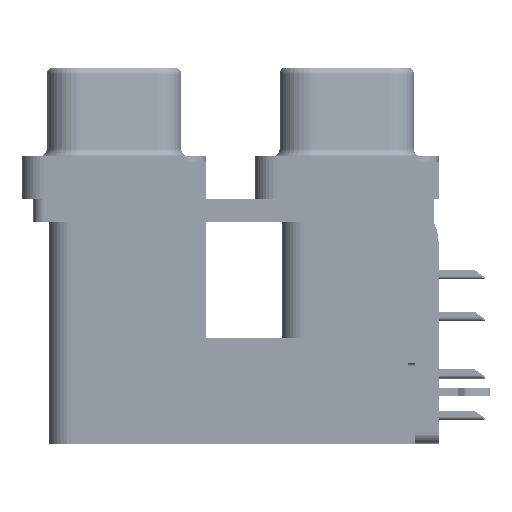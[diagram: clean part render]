
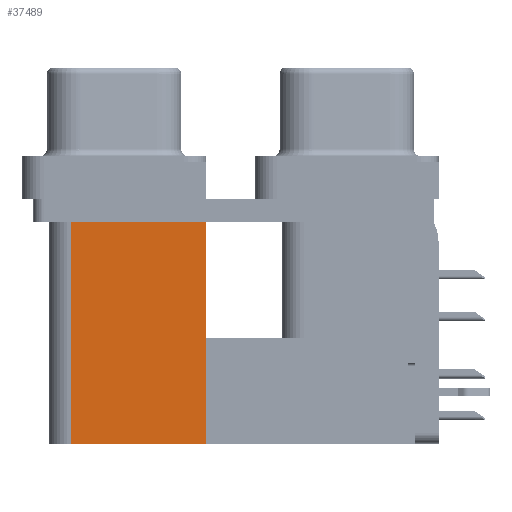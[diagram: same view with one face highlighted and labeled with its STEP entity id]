
A CAD part, left-side view. The second image highlights one B-rep face of the part: STEP entity #37489.
In plain terms, the highlighted planar face has unit normal (-1, 0, 0).
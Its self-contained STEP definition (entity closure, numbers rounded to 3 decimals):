
#683 = DIRECTION ( 'NONE',  ( 0., 1., 0. ) ) ;
#1632 = VECTOR ( 'NONE', #683, 1000. ) ;
#2077 = LINE ( 'NONE', #22358, #21959 ) ;
#6823 = ORIENTED_EDGE ( 'NONE', *, *, #8162, .T. ) ;
#7045 = EDGE_CURVE ( 'NONE', #44615, #36354, #29477, .T. ) ;
#8162 = EDGE_CURVE ( 'NONE', #44615, #46907, #8947, .T. ) ;
#8218 = CARTESIAN_POINT ( 'NONE',  ( 3.79, 9.6, -19.2 ) ) ;
#8947 = LINE ( 'NONE', #44654, #21041 ) ;
#10580 = CARTESIAN_POINT ( 'NONE',  ( 3.79, 18.8, -19.2 ) ) ;
#11832 = AXIS2_PLACEMENT_3D ( 'NONE', #8218, #40719, #20476 ) ;
#12239 = FACE_OUTER_BOUND ( 'NONE', #30949, .T. ) ;
#14027 = CARTESIAN_POINT ( 'NONE',  ( 3.79, 9.6, -19.2 ) ) ;
#14357 = ORIENTED_EDGE ( 'NONE', *, *, #27349, .F. ) ;
#18900 = DIRECTION ( 'NONE',  ( 0., 0., 1. ) ) ;
#19880 = DIRECTION ( 'NONE',  ( 0., 1., 0. ) ) ;
#20476 = DIRECTION ( 'NONE',  ( 0., 0., -1. ) ) ;
#21041 = VECTOR ( 'NONE', #24153, 1000. ) ;
#21281 = ORIENTED_EDGE ( 'NONE', *, *, #7045, .F. ) ;
#21959 = VECTOR ( 'NONE', #18900, 1000. ) ;
#22358 = CARTESIAN_POINT ( 'NONE',  ( 3.79, 18.8, -19.2 ) ) ;
#24153 = DIRECTION ( 'NONE',  ( 0., 0., 1. ) ) ;
#27349 = EDGE_CURVE ( 'NONE', #36354, #45209, #2077, .T. ) ;
#27851 = EDGE_CURVE ( 'NONE', #46907, #45209, #49165, .T. ) ;
#28479 = PLANE ( 'NONE',  #11832 ) ;
#29477 = LINE ( 'NONE', #14027, #1632 ) ;
#30949 = EDGE_LOOP ( 'NONE', ( #37202, #14357, #21281, #6823 ) ) ;
#35881 = CARTESIAN_POINT ( 'NONE',  ( 3.79, 9.6, -19.2 ) ) ;
#36354 = VERTEX_POINT ( 'NONE', #10580 ) ;
#37202 = ORIENTED_EDGE ( 'NONE', *, *, #27851, .T. ) ;
#37489 = ADVANCED_FACE ( 'NONE', ( #12239 ), #28479, .F. ) ;
#37788 = CARTESIAN_POINT ( 'NONE',  ( 3.79, 9.6, -2.5 ) ) ;
#40719 = DIRECTION ( 'NONE',  ( 1., 0., 0. ) ) ;
#40855 = CARTESIAN_POINT ( 'NONE',  ( 3.79, 18.8, -2.5 ) ) ;
#43852 = CARTESIAN_POINT ( 'NONE',  ( 3.79, 9.6, -2.5 ) ) ;
#44615 = VERTEX_POINT ( 'NONE', #35881 ) ;
#44654 = CARTESIAN_POINT ( 'NONE',  ( 3.79, 9.6, -19.2 ) ) ;
#45209 = VERTEX_POINT ( 'NONE', #40855 ) ;
#46907 = VERTEX_POINT ( 'NONE', #37788 ) ;
#49165 = LINE ( 'NONE', #43852, #50786 ) ;
#50786 = VECTOR ( 'NONE', #19880, 1000. ) ;
